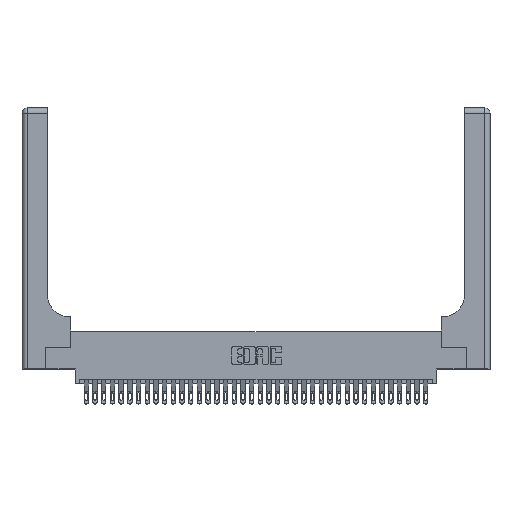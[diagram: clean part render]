
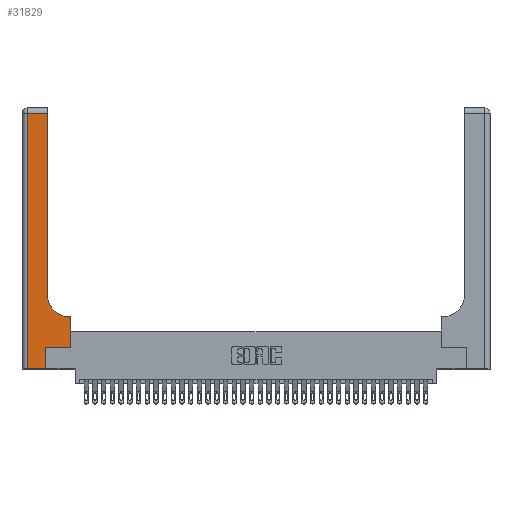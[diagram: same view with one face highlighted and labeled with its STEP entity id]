
A CAD part, top view. The second image highlights one B-rep face of the part: STEP entity #31829.
In plain terms, the highlighted planar face has unit normal (0, 0, 1).
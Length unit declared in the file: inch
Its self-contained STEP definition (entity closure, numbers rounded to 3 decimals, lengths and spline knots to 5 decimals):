
#230 = CARTESIAN_POINT ( 'NONE',  ( 0., 0., 0.37 ) ) ;
#247 = FACE_OUTER_BOUND ( 'NONE', #1119, .T. ) ;
#507 = CARTESIAN_POINT ( 'NONE',  ( 0.5415, 0.85, 0.37 ) ) ;
#798 = VECTOR ( 'NONE', #33252, 39.37008 ) ;
#1119 = EDGE_LOOP ( 'NONE', ( #31364, #1622, #11100, #34047, #12901, #28241, #21458, #16488, #31845 ) ) ;
#1544 = VECTOR ( 'NONE', #35180, 39.37008 ) ;
#1622 = ORIENTED_EDGE ( 'NONE', *, *, #21297, .T. ) ;
#1983 = VERTEX_POINT ( 'NONE', #23183 ) ;
#2306 = VERTEX_POINT ( 'NONE', #9967 ) ;
#3431 = DIRECTION ( 'NONE',  ( 1., 0., 0. ) ) ;
#3819 = VECTOR ( 'NONE', #30576, 39.37008 ) ;
#4008 = LINE ( 'NONE', #230, #10767 ) ;
#5178 = EDGE_CURVE ( 'NONE', #21637, #19258, #7600, .T. ) ;
#5564 = EDGE_CURVE ( 'NONE', #35755, #2306, #4008, .T. ) ;
#5587 = VERTEX_POINT ( 'NONE', #23413 ) ;
#5809 = AXIS2_PLACEMENT_3D ( 'NONE', #12181, #32332, #15039 ) ;
#7600 = LINE ( 'NONE', #13125, #798 ) ;
#9268 = CARTESIAN_POINT ( 'NONE',  ( 0.06, 3., 0.37 ) ) ;
#9804 = AXIS2_PLACEMENT_3D ( 'NONE', #507, #20664, #3431 ) ;
#9967 = CARTESIAN_POINT ( 'NONE',  ( 0.269, 0., 0.37 ) ) ;
#10767 = VECTOR ( 'NONE', #28979, 39.37008 ) ;
#11100 = ORIENTED_EDGE ( 'NONE', *, *, #17456, .T. ) ;
#11476 = LINE ( 'NONE', #21854, #3819 ) ;
#11735 = VERTEX_POINT ( 'NONE', #35191 ) ;
#11788 = VECTOR ( 'NONE', #23971, 39.37008 ) ;
#12181 = CARTESIAN_POINT ( 'NONE',  ( 0., 3., 0.37 ) ) ;
#12413 = CARTESIAN_POINT ( 'NONE',  ( 0.269, 0., 0.37 ) ) ;
#12670 = DIRECTION ( 'NONE',  ( -1., 0., 0. ) ) ;
#12901 = ORIENTED_EDGE ( 'NONE', *, *, #35656, .T. ) ;
#13125 = CARTESIAN_POINT ( 'NONE',  ( 0.5585, 0.25, 0.37 ) ) ;
#14103 = DIRECTION ( 'NONE',  ( -1., 0., 0. ) ) ;
#15039 = DIRECTION ( 'NONE',  ( -1., 0., 0. ) ) ;
#16259 = EDGE_CURVE ( 'NONE', #1983, #5587, #33993, .T. ) ;
#16488 = ORIENTED_EDGE ( 'NONE', *, *, #18407, .T. ) ;
#16831 = LINE ( 'NONE', #9268, #1544 ) ;
#17456 = EDGE_CURVE ( 'NONE', #36414, #35755, #16831, .T. ) ;
#18401 = VERTEX_POINT ( 'NONE', #29922 ) ;
#18407 = EDGE_CURVE ( 'NONE', #19258, #1983, #22647, .T. ) ;
#18426 = CARTESIAN_POINT ( 'NONE',  ( 0.2915, 0.6, 0.37 ) ) ;
#19258 = VERTEX_POINT ( 'NONE', #24694 ) ;
#19430 = LINE ( 'NONE', #12413, #11788 ) ;
#20664 = DIRECTION ( 'NONE',  ( 0., 0., -1. ) ) ;
#20733 = PLANE ( 'NONE',  #5809 ) ;
#21030 = VECTOR ( 'NONE', #14103, 39.37008 ) ;
#21297 = EDGE_CURVE ( 'NONE', #11735, #36414, #28724, .T. ) ;
#21458 = ORIENTED_EDGE ( 'NONE', *, *, #5178, .T. ) ;
#21543 = CARTESIAN_POINT ( 'NONE',  ( 0.06, 2.94, 0.37 ) ) ;
#21637 = VERTEX_POINT ( 'NONE', #27097 ) ;
#21854 = CARTESIAN_POINT ( 'NONE',  ( 0.2915, 3., 0.37 ) ) ;
#22647 = LINE ( 'NONE', #18426, #24443 ) ;
#22803 = CARTESIAN_POINT ( 'NONE',  ( 0., 2.94, 0.37 ) ) ;
#23183 = CARTESIAN_POINT ( 'NONE',  ( 0.5415, 0.6, 0.37 ) ) ;
#23413 = CARTESIAN_POINT ( 'NONE',  ( 0.2915, 0.85, 0.37 ) ) ;
#23971 = DIRECTION ( 'NONE',  ( 0., 1., 0. ) ) ;
#24443 = VECTOR ( 'NONE', #12670, 39.37008 ) ;
#24694 = CARTESIAN_POINT ( 'NONE',  ( 0.5585, 0.6, 0.37 ) ) ;
#27097 = CARTESIAN_POINT ( 'NONE',  ( 0.5585, 0.25, 0.37 ) ) ;
#28241 = ORIENTED_EDGE ( 'NONE', *, *, #28727, .T. ) ;
#28724 = LINE ( 'NONE', #22803, #21030 ) ;
#28727 = EDGE_CURVE ( 'NONE', #18401, #21637, #36052, .T. ) ;
#28979 = DIRECTION ( 'NONE',  ( 1., 0., 0. ) ) ;
#29922 = CARTESIAN_POINT ( 'NONE',  ( 0.269, 0.25, 0.37 ) ) ;
#30012 = DIRECTION ( 'NONE',  ( 1., 0., 0. ) ) ;
#30576 = DIRECTION ( 'NONE',  ( 0., 1., 0. ) ) ;
#31364 = ORIENTED_EDGE ( 'NONE', *, *, #32638, .T. ) ;
#31829 = ADVANCED_FACE ( 'NONE', ( #247 ), #20733, .F. ) ;
#31845 = ORIENTED_EDGE ( 'NONE', *, *, #16259, .T. ) ;
#32332 = DIRECTION ( 'NONE',  ( 0., 0., -1. ) ) ;
#32638 = EDGE_CURVE ( 'NONE', #5587, #11735, #11476, .T. ) ;
#32876 = CARTESIAN_POINT ( 'NONE',  ( 0.269, 0.25, 0.37 ) ) ;
#33035 = CARTESIAN_POINT ( 'NONE',  ( 0.06, 0., 0.37 ) ) ;
#33252 = DIRECTION ( 'NONE',  ( 0., 1., 0. ) ) ;
#33993 = CIRCLE ( 'NONE', #9804, 0.25 ) ;
#34047 = ORIENTED_EDGE ( 'NONE', *, *, #5564, .T. ) ;
#35146 = VECTOR ( 'NONE', #30012, 39.37008 ) ;
#35180 = DIRECTION ( 'NONE',  ( 0., -1., 0. ) ) ;
#35191 = CARTESIAN_POINT ( 'NONE',  ( 0.2915, 2.94, 0.37 ) ) ;
#35656 = EDGE_CURVE ( 'NONE', #2306, #18401, #19430, .T. ) ;
#35755 = VERTEX_POINT ( 'NONE', #33035 ) ;
#36052 = LINE ( 'NONE', #32876, #35146 ) ;
#36414 = VERTEX_POINT ( 'NONE', #21543 ) ;
